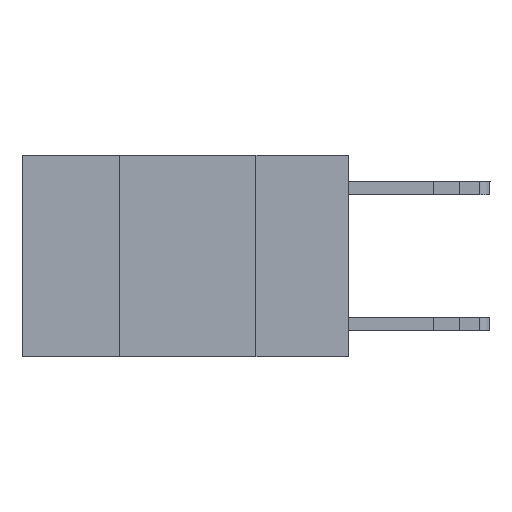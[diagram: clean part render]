
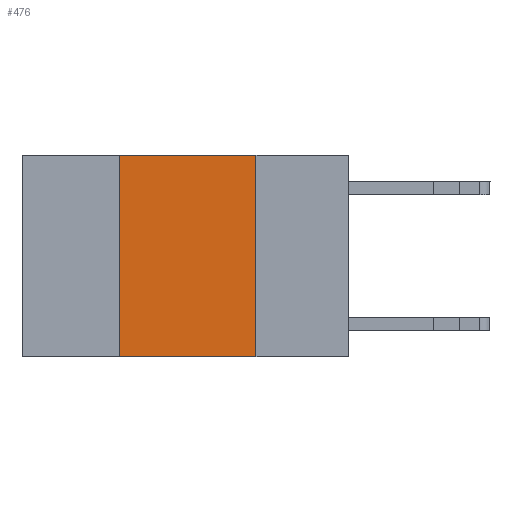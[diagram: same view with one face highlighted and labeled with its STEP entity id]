
A CAD part, left-side view. The second image highlights one B-rep face of the part: STEP entity #476.
In plain terms, the highlighted planar face has unit normal (-1, 0, 0).
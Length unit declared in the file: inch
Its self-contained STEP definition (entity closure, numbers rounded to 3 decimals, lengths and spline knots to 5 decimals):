
#126 = CARTESIAN_POINT ( 'NONE',  ( 0., 0.6, -0.37 ) ) ;
#476 = ADVANCED_FACE ( 'NONE', ( #14357 ), #7675, .F. ) ;
#1094 = DIRECTION ( 'NONE',  ( 0., 0., -1. ) ) ;
#2446 = VERTEX_POINT ( 'NONE', #14698 ) ;
#2677 = CARTESIAN_POINT ( 'NONE',  ( 0., 0.42, 0. ) ) ;
#2781 = CARTESIAN_POINT ( 'NONE',  ( 0., 0.42, 0. ) ) ;
#3001 = DIRECTION ( 'NONE',  ( 0., 0., -1. ) ) ;
#3711 = ORIENTED_EDGE ( 'NONE', *, *, #8078, .T. ) ;
#3845 = LINE ( 'NONE', #2677, #13127 ) ;
#4931 = VECTOR ( 'NONE', #15102, 39.37008 ) ;
#5563 = LINE ( 'NONE', #126, #14998 ) ;
#5588 = EDGE_CURVE ( 'NONE', #9718, #2446, #11121, .T. ) ;
#5799 = CARTESIAN_POINT ( 'NONE',  ( 0., 0.6, 0. ) ) ;
#5964 = CARTESIAN_POINT ( 'NONE',  ( 0., 0.17, -0.37 ) ) ;
#6113 = ORIENTED_EDGE ( 'NONE', *, *, #11962, .F. ) ;
#7675 = PLANE ( 'NONE',  #12734 ) ;
#8078 = EDGE_CURVE ( 'NONE', #11060, #10157, #5563, .T. ) ;
#8410 = DIRECTION ( 'NONE',  ( 0., -1., 0. ) ) ;
#8522 = VECTOR ( 'NONE', #1094, 39.37008 ) ;
#8844 = CARTESIAN_POINT ( 'NONE',  ( 0., 0.6, 0. ) ) ;
#8881 = LINE ( 'NONE', #9320, #8522 ) ;
#9017 = EDGE_LOOP ( 'NONE', ( #6113, #9194, #12659, #3711 ) ) ;
#9194 = ORIENTED_EDGE ( 'NONE', *, *, #5588, .F. ) ;
#9320 = CARTESIAN_POINT ( 'NONE',  ( 0., 0.17, 0. ) ) ;
#9652 = EDGE_CURVE ( 'NONE', #11060, #9718, #3845, .T. ) ;
#9718 = VERTEX_POINT ( 'NONE', #2781 ) ;
#10034 = DIRECTION ( 'NONE',  ( 1., 0., 0. ) ) ;
#10157 = VERTEX_POINT ( 'NONE', #5964 ) ;
#10877 = DIRECTION ( 'NONE',  ( 0., 0., 1. ) ) ;
#10989 = CARTESIAN_POINT ( 'NONE',  ( 0., 0.42, -0.37 ) ) ;
#11060 = VERTEX_POINT ( 'NONE', #10989 ) ;
#11121 = LINE ( 'NONE', #5799, #4931 ) ;
#11962 = EDGE_CURVE ( 'NONE', #2446, #10157, #8881, .T. ) ;
#12659 = ORIENTED_EDGE ( 'NONE', *, *, #9652, .F. ) ;
#12734 = AXIS2_PLACEMENT_3D ( 'NONE', #8844, #10034, #3001 ) ;
#13127 = VECTOR ( 'NONE', #10877, 39.37008 ) ;
#14357 = FACE_OUTER_BOUND ( 'NONE', #9017, .T. ) ;
#14698 = CARTESIAN_POINT ( 'NONE',  ( 0., 0.17, 0. ) ) ;
#14998 = VECTOR ( 'NONE', #8410, 39.37008 ) ;
#15102 = DIRECTION ( 'NONE',  ( 0., -1., 0. ) ) ;
